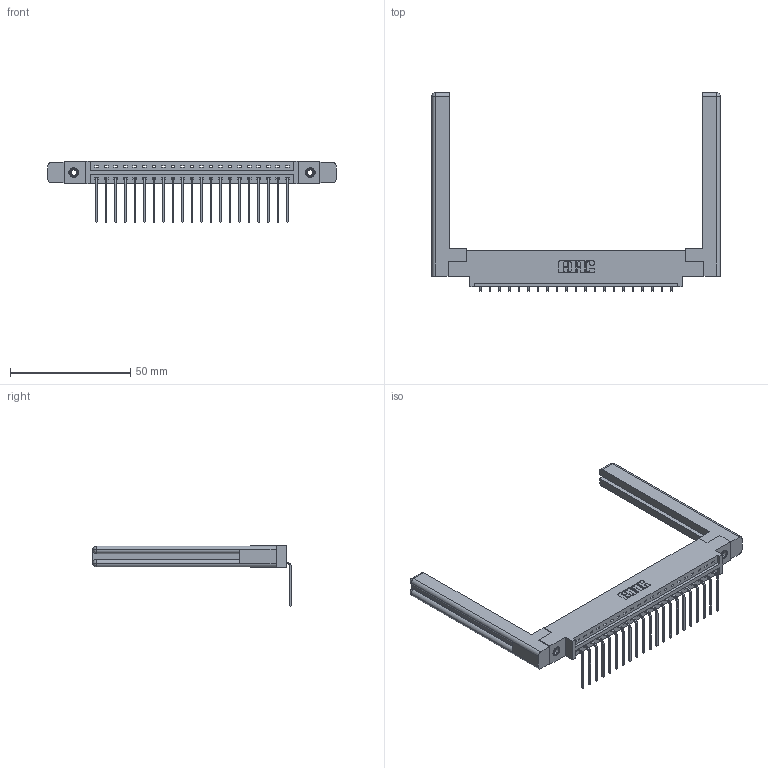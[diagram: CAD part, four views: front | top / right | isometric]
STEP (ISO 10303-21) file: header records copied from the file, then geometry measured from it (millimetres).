
FILE_DESCRIPTION (( 'STEP AP203' ), '1' );
FILE_NAME ('337-021-559-658.STEP', '2019-09-29T01:20:14', ( '' ), ( '' ), 'SwSTEP 2.0', 'SolidWorks 2016', '' );
FILE_SCHEMA (( 'CONFIG_CONTROL_DESIGN' ));
Length unit declared in the file: inch
Products named in the file (5): 307-220-058; 345-250-001_345-250-001-102; 337 Part_0.170 Offset - 0.156 Dia-TI; 345-292-001_558 559 Tail - 1; 337-021-559-658
Assembly tree (26 placements, depth 2):
  337-021-559-658
    337 Part_0.170 Offset - 0.156 Dia-TI
    345-292-001_558 559 Tail - 1  x21
    345-250-001_345-250-001-102  x2
    307-220-058  x2
Bounding box: 119.84 x 82.49 x 25.53 mm (x, y, z)
Volume: 19306.9 mm3; surface area: 18172.5 mm2
Topology: 26 solids, 26 shells, 1604 faces, 4751 edges, 3126 vertices
Faces by surface type: plane 1166, cylinder 414, cone 12, torus 12
Entity records: 21176 total; most frequent: CARTESIAN_POINT 3688, ORIENTED_EDGE 3584, DIRECTION 3166, EDGE_CURVE 1792, LINE 1616, VECTOR 1616, VERTEX_POINT 1186, AXIS2_PLACEMENT_3D 775
